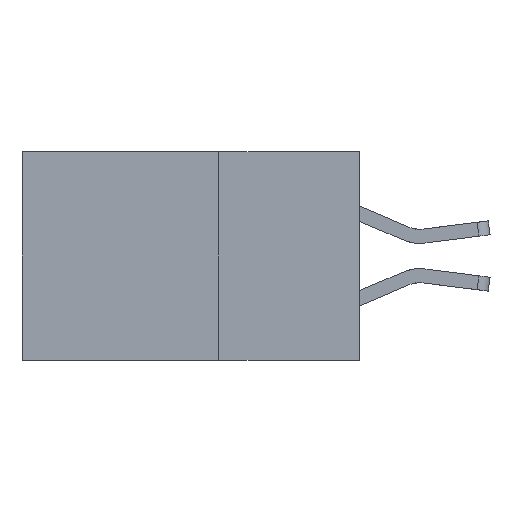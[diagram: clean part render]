
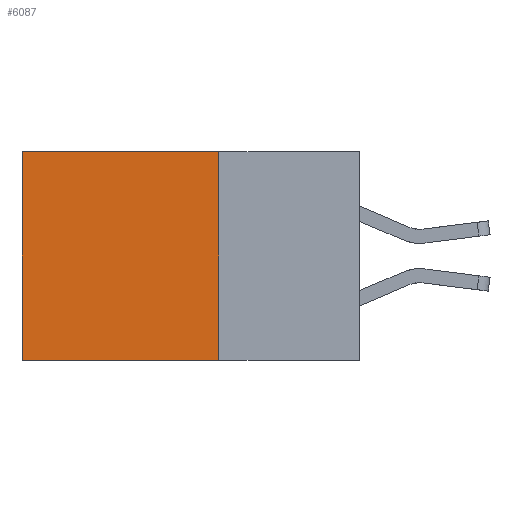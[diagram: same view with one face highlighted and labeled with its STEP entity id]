
A CAD part, left-side view. The second image highlights one B-rep face of the part: STEP entity #6087.
In plain terms, the highlighted planar face has unit normal (-1, 0, 0).
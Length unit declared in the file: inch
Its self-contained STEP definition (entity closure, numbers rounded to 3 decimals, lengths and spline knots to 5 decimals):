
#72 = CARTESIAN_POINT ( 'NONE',  ( 0.2875, 0.25, 0. ) ) ;
#607 = EDGE_CURVE ( 'NONE', #7139, #4622, #9699, .T. ) ;
#682 = EDGE_CURVE ( 'NONE', #4420, #7139, #9482, .T. ) ;
#2497 = VECTOR ( 'NONE', #5181, 39.37008 ) ;
#3169 = CARTESIAN_POINT ( 'NONE',  ( 0.2875, 0.6, 0. ) ) ;
#3789 = FACE_OUTER_BOUND ( 'NONE', #8591, .T. ) ;
#4411 = LINE ( 'NONE', #7406, #2497 ) ;
#4420 = VERTEX_POINT ( 'NONE', #72 ) ;
#4622 = VERTEX_POINT ( 'NONE', #7326 ) ;
#4912 = CARTESIAN_POINT ( 'NONE',  ( 0.2875, 0.25, 0. ) ) ;
#4923 = PLANE ( 'NONE',  #6988 ) ;
#4964 = DIRECTION ( 'NONE',  ( 0., 0., -1. ) ) ;
#5090 = CARTESIAN_POINT ( 'NONE',  ( 0.2875, 0.6, 0. ) ) ;
#5181 = DIRECTION ( 'NONE',  ( 0., 1., 0. ) ) ;
#5772 = DIRECTION ( 'NONE',  ( 0., 0., -1. ) ) ;
#5985 = ORIENTED_EDGE ( 'NONE', *, *, #607, .T. ) ;
#6068 = CARTESIAN_POINT ( 'NONE',  ( 0.2875, 0.25, 0. ) ) ;
#6087 = ADVANCED_FACE ( 'NONE', ( #3789 ), #4923, .F. ) ;
#6143 = DIRECTION ( 'NONE',  ( 0., 0., -1. ) ) ;
#6152 = ORIENTED_EDGE ( 'NONE', *, *, #8031, .F. ) ;
#6154 = DIRECTION ( 'NONE',  ( 1., 0., 0. ) ) ;
#6156 = VECTOR ( 'NONE', #4964, 39.37008 ) ;
#6397 = ORIENTED_EDGE ( 'NONE', *, *, #7000, .F. ) ;
#6702 = VECTOR ( 'NONE', #6993, 39.37008 ) ;
#6892 = ORIENTED_EDGE ( 'NONE', *, *, #682, .T. ) ;
#6983 = CARTESIAN_POINT ( 'NONE',  ( 0.2875, 0.25, -0.37 ) ) ;
#6988 = AXIS2_PLACEMENT_3D ( 'NONE', #4912, #6154, #6143 ) ;
#6993 = DIRECTION ( 'NONE',  ( 0., 1., 0. ) ) ;
#7000 = EDGE_CURVE ( 'NONE', #4420, #7537, #8104, .T. ) ;
#7139 = VERTEX_POINT ( 'NONE', #5090 ) ;
#7212 = CARTESIAN_POINT ( 'NONE',  ( 0.2875, 0.25, 0. ) ) ;
#7326 = CARTESIAN_POINT ( 'NONE',  ( 0.2875, 0.6, -0.37 ) ) ;
#7406 = CARTESIAN_POINT ( 'NONE',  ( 0.2875, 0.25, -0.37 ) ) ;
#7537 = VERTEX_POINT ( 'NONE', #6983 ) ;
#7850 = VECTOR ( 'NONE', #5772, 39.37008 ) ;
#8031 = EDGE_CURVE ( 'NONE', #7537, #4622, #4411, .T. ) ;
#8104 = LINE ( 'NONE', #7212, #6156 ) ;
#8591 = EDGE_LOOP ( 'NONE', ( #5985, #6152, #6397, #6892 ) ) ;
#9482 = LINE ( 'NONE', #6068, #6702 ) ;
#9699 = LINE ( 'NONE', #3169, #7850 ) ;
